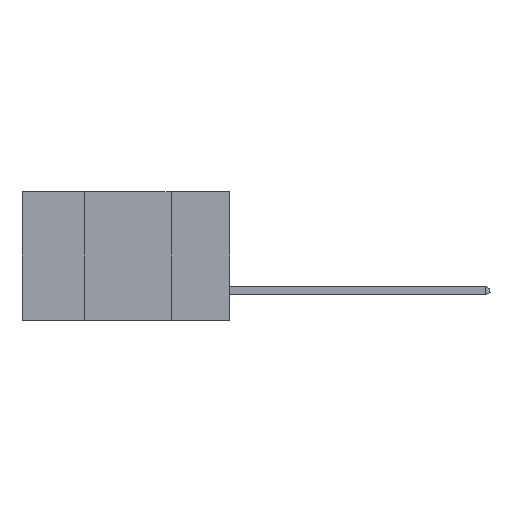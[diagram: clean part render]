
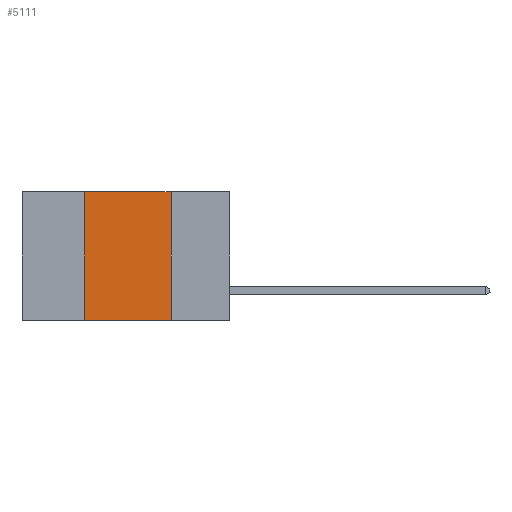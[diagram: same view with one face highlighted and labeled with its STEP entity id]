
A CAD part, left-side view. The second image highlights one B-rep face of the part: STEP entity #5111.
In plain terms, the highlighted planar face has unit normal (-1, 0, 0).
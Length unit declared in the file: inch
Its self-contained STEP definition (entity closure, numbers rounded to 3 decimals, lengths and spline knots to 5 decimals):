
#146 = CARTESIAN_POINT ( 'NONE',  ( 0., 0.17, 0. ) ) ;
#379 = DIRECTION ( 'NONE',  ( 1., 0., 0. ) ) ;
#451 = DIRECTION ( 'NONE',  ( 0., -1., 0. ) ) ;
#1691 = VERTEX_POINT ( 'NONE', #146 ) ;
#1989 = LINE ( 'NONE', #2642, #9477 ) ;
#2250 = CARTESIAN_POINT ( 'NONE',  ( 0., 0.42, 0. ) ) ;
#2569 = CARTESIAN_POINT ( 'NONE',  ( 0., 0.17, 0. ) ) ;
#2642 = CARTESIAN_POINT ( 'NONE',  ( 0., 0.6, 0. ) ) ;
#3475 = CARTESIAN_POINT ( 'NONE',  ( 0., 0.6, -0.37 ) ) ;
#3945 = CARTESIAN_POINT ( 'NONE',  ( 0., 0.6, 0. ) ) ;
#4291 = ORIENTED_EDGE ( 'NONE', *, *, #13976, .T. ) ;
#4310 = VECTOR ( 'NONE', #10611, 39.37008 ) ;
#4817 = DIRECTION ( 'NONE',  ( 0., -1., 0. ) ) ;
#5055 = LINE ( 'NONE', #2250, #4310 ) ;
#5111 = ADVANCED_FACE ( 'NONE', ( #12299 ), #13414, .F. ) ;
#6123 = EDGE_CURVE ( 'NONE', #8295, #1691, #1989, .T. ) ;
#6158 = VECTOR ( 'NONE', #4817, 39.37008 ) ;
#6975 = ORIENTED_EDGE ( 'NONE', *, *, #8333, .F. ) ;
#7677 = AXIS2_PLACEMENT_3D ( 'NONE', #3945, #379, #12268 ) ;
#7739 = ORIENTED_EDGE ( 'NONE', *, *, #6123, .F. ) ;
#8295 = VERTEX_POINT ( 'NONE', #11827 ) ;
#8333 = EDGE_CURVE ( 'NONE', #1691, #9383, #12180, .T. ) ;
#9003 = CARTESIAN_POINT ( 'NONE',  ( 0., 0.17, -0.37 ) ) ;
#9010 = VECTOR ( 'NONE', #12026, 39.37008 ) ;
#9383 = VERTEX_POINT ( 'NONE', #9003 ) ;
#9477 = VECTOR ( 'NONE', #451, 39.37008 ) ;
#10068 = VERTEX_POINT ( 'NONE', #11381 ) ;
#10472 = LINE ( 'NONE', #3475, #6158 ) ;
#10611 = DIRECTION ( 'NONE',  ( 0., 0., 1. ) ) ;
#11381 = CARTESIAN_POINT ( 'NONE',  ( 0., 0.42, -0.37 ) ) ;
#11827 = CARTESIAN_POINT ( 'NONE',  ( 0., 0.42, 0. ) ) ;
#12026 = DIRECTION ( 'NONE',  ( 0., 0., -1. ) ) ;
#12180 = LINE ( 'NONE', #2569, #9010 ) ;
#12268 = DIRECTION ( 'NONE',  ( 0., 0., -1. ) ) ;
#12299 = FACE_OUTER_BOUND ( 'NONE', #12531, .T. ) ;
#12531 = EDGE_LOOP ( 'NONE', ( #6975, #7739, #14980, #4291 ) ) ;
#13414 = PLANE ( 'NONE',  #7677 ) ;
#13930 = EDGE_CURVE ( 'NONE', #10068, #8295, #5055, .T. ) ;
#13976 = EDGE_CURVE ( 'NONE', #10068, #9383, #10472, .T. ) ;
#14980 = ORIENTED_EDGE ( 'NONE', *, *, #13930, .F. ) ;
